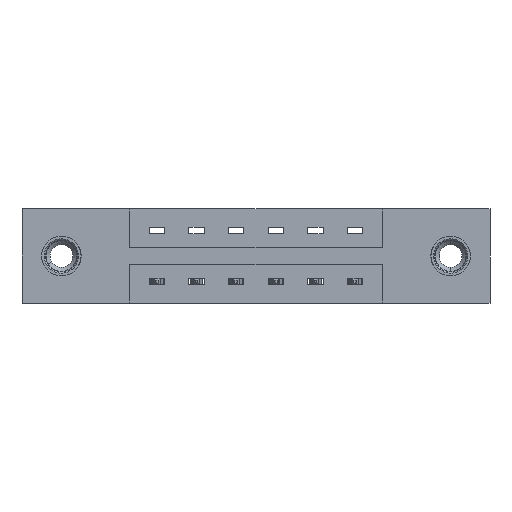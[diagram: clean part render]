
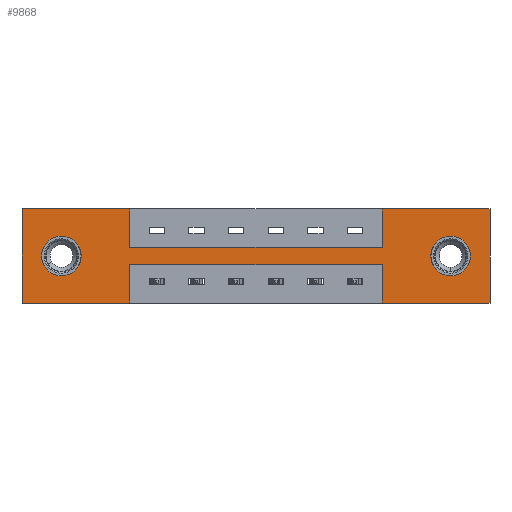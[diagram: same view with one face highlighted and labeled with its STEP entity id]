
A CAD part, front view. The second image highlights one B-rep face of the part: STEP entity #9868.
In plain terms, the highlighted planar face has unit normal (0, -1, 0).
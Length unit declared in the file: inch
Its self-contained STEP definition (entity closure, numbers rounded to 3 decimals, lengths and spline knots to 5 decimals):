
#16 = EDGE_CURVE ( 'NONE', #8204, #5925, #8514, .T. ) ;
#119 = DIRECTION ( 'NONE',  ( 0., 0., -1. ) ) ;
#130 = VERTEX_POINT ( 'NONE', #5805 ) ;
#189 = ORIENTED_EDGE ( 'NONE', *, *, #2319, .F. ) ;
#256 = DIRECTION ( 'NONE',  ( 0., 0., -1. ) ) ;
#269 = LINE ( 'NONE', #8182, #2256 ) ;
#465 = ORIENTED_EDGE ( 'NONE', *, *, #6879, .F. ) ;
#544 = AXIS2_PLACEMENT_3D ( 'NONE', #9028, #4375, #9754 ) ;
#551 = VERTEX_POINT ( 'NONE', #1400 ) ;
#689 = EDGE_LOOP ( 'NONE', ( #8340, #10272, #4398, #189, #2454, #465, #2722, #9022, #719, #7249, #9243, #988 ) ) ;
#719 = ORIENTED_EDGE ( 'NONE', *, *, #2528, .F. ) ;
#733 = LINE ( 'NONE', #8028, #8801 ) ;
#818 = VERTEX_POINT ( 'NONE', #6511 ) ;
#921 = VERTEX_POINT ( 'NONE', #7230 ) ;
#923 = PLANE ( 'NONE',  #8842 ) ;
#988 = ORIENTED_EDGE ( 'NONE', *, *, #16, .F. ) ;
#1034 = DIRECTION ( 'NONE',  ( 0., 1., 0. ) ) ;
#1042 = DIRECTION ( 'NONE',  ( 1., 0., 0. ) ) ;
#1070 = LINE ( 'NONE', #3638, #7321 ) ;
#1096 = DIRECTION ( 'NONE',  ( 0., 0., -1. ) ) ;
#1184 = CARTESIAN_POINT ( 'NONE',  ( 0.425, 0., -0.15 ) ) ;
#1239 = EDGE_CURVE ( 'NONE', #4260, #7239, #8824, .T. ) ;
#1400 = CARTESIAN_POINT ( 'NONE',  ( 0.155, 0., -0.107 ) ) ;
#1656 = DIRECTION ( 'NONE',  ( 0., 0., -1. ) ) ;
#1666 = EDGE_LOOP ( 'NONE', ( #8105, #7600 ) ) ;
#1670 = VECTOR ( 'NONE', #256, 39.37008 ) ;
#1675 = AXIS2_PLACEMENT_3D ( 'NONE', #5954, #1034, #6764 ) ;
#1773 = DIRECTION ( 'NONE',  ( 0., 0., -1. ) ) ;
#1866 = CARTESIAN_POINT ( 'NONE',  ( 1.842, 0., 0. ) ) ;
#1872 = VECTOR ( 'NONE', #8496, 39.37008 ) ;
#1880 = DIRECTION ( 'NONE',  ( 0., 0., -1. ) ) ;
#1893 = CARTESIAN_POINT ( 'NONE',  ( 0., 0., -0.37 ) ) ;
#2256 = VECTOR ( 'NONE', #4251, 39.37008 ) ;
#2319 = EDGE_CURVE ( 'NONE', #818, #4869, #4918, .T. ) ;
#2454 = ORIENTED_EDGE ( 'NONE', *, *, #5068, .F. ) ;
#2528 = EDGE_CURVE ( 'NONE', #7880, #9551, #7389, .T. ) ;
#2550 = CARTESIAN_POINT ( 'NONE',  ( 0.425, 0., -0.22 ) ) ;
#2722 = ORIENTED_EDGE ( 'NONE', *, *, #4743, .F. ) ;
#2820 = CARTESIAN_POINT ( 'NONE',  ( 0., 0., 0. ) ) ;
#2867 = CIRCLE ( 'NONE', #5391, 0.078 ) ;
#2907 = CARTESIAN_POINT ( 'NONE',  ( 0.425, 0., 0. ) ) ;
#2940 = CARTESIAN_POINT ( 'NONE',  ( 1.417, 0., 0. ) ) ;
#3068 = DIRECTION ( 'NONE',  ( -1., 0., 0. ) ) ;
#3164 = EDGE_CURVE ( 'NONE', #8799, #7880, #10157, .T. ) ;
#3201 = LINE ( 'NONE', #10294, #5108 ) ;
#3638 = CARTESIAN_POINT ( 'NONE',  ( 1.417, 0., -0.37 ) ) ;
#3680 = EDGE_CURVE ( 'NONE', #9551, #921, #4774, .T. ) ;
#3857 = CIRCLE ( 'NONE', #544, 0.078 ) ;
#3888 = CARTESIAN_POINT ( 'NONE',  ( 0.155, 0., -0.263 ) ) ;
#4101 = FACE_BOUND ( 'NONE', #8765, .T. ) ;
#4143 = VERTEX_POINT ( 'NONE', #10268 ) ;
#4235 = DIRECTION ( 'NONE',  ( -1., 0., 0. ) ) ;
#4251 = DIRECTION ( 'NONE',  ( -1., 0., 0. ) ) ;
#4260 = VERTEX_POINT ( 'NONE', #4265 ) ;
#4265 = CARTESIAN_POINT ( 'NONE',  ( 1.687, 0., -0.263 ) ) ;
#4375 = DIRECTION ( 'NONE',  ( 0., 1., 0. ) ) ;
#4398 = ORIENTED_EDGE ( 'NONE', *, *, #5270, .F. ) ;
#4439 = CARTESIAN_POINT ( 'NONE',  ( 0.425, 0., 0. ) ) ;
#4598 = FACE_BOUND ( 'NONE', #1666, .T. ) ;
#4679 = LINE ( 'NONE', #5234, #1670 ) ;
#4743 = EDGE_CURVE ( 'NONE', #921, #4143, #5968, .T. ) ;
#4774 = LINE ( 'NONE', #8308, #8216 ) ;
#4869 = VERTEX_POINT ( 'NONE', #5518 ) ;
#4918 = LINE ( 'NONE', #5027, #8817 ) ;
#5027 = CARTESIAN_POINT ( 'NONE',  ( 0., 0., -0.37 ) ) ;
#5068 = EDGE_CURVE ( 'NONE', #8458, #818, #3201, .T. ) ;
#5108 = VECTOR ( 'NONE', #1656, 39.37008 ) ;
#5120 = DIRECTION ( 'NONE',  ( 0., 1., 0. ) ) ;
#5234 = CARTESIAN_POINT ( 'NONE',  ( 0.425, 0., -0.37 ) ) ;
#5270 = EDGE_CURVE ( 'NONE', #4869, #130, #1070, .T. ) ;
#5391 = AXIS2_PLACEMENT_3D ( 'NONE', #9713, #5120, #119 ) ;
#5477 = VERTEX_POINT ( 'NONE', #3888 ) ;
#5518 = CARTESIAN_POINT ( 'NONE',  ( 1.417, 0., -0.37 ) ) ;
#5701 = CIRCLE ( 'NONE', #1675, 0.078 ) ;
#5785 = EDGE_CURVE ( 'NONE', #130, #8848, #269, .T. ) ;
#5805 = CARTESIAN_POINT ( 'NONE',  ( 1.417, 0., -0.22 ) ) ;
#5925 = VERTEX_POINT ( 'NONE', #1893 ) ;
#5939 = AXIS2_PLACEMENT_3D ( 'NONE', #9605, #6271, #1880 ) ;
#5954 = CARTESIAN_POINT ( 'NONE',  ( 0.155, 0., -0.185 ) ) ;
#5968 = LINE ( 'NONE', #2940, #1872 ) ;
#6022 = VECTOR ( 'NONE', #7617, 39.37008 ) ;
#6063 = ORIENTED_EDGE ( 'NONE', *, *, #7382, .T. ) ;
#6144 = VECTOR ( 'NONE', #8409, 39.37008 ) ;
#6246 = ORIENTED_EDGE ( 'NONE', *, *, #1239, .T. ) ;
#6271 = DIRECTION ( 'NONE',  ( 0., 1., 0. ) ) ;
#6434 = VECTOR ( 'NONE', #3068, 39.37008 ) ;
#6511 = CARTESIAN_POINT ( 'NONE',  ( 1.842, 0., -0.37 ) ) ;
#6656 = DIRECTION ( 'NONE',  ( 0., -1., 0. ) ) ;
#6764 = DIRECTION ( 'NONE',  ( 0., 0., 1. ) ) ;
#6862 = EDGE_CURVE ( 'NONE', #8848, #8204, #4679, .T. ) ;
#6879 = EDGE_CURVE ( 'NONE', #4143, #8458, #9835, .T. ) ;
#7197 = EDGE_CURVE ( 'NONE', #5925, #8799, #733, .T. ) ;
#7230 = CARTESIAN_POINT ( 'NONE',  ( 1.417, 0., -0.15 ) ) ;
#7239 = VERTEX_POINT ( 'NONE', #10258 ) ;
#7249 = ORIENTED_EDGE ( 'NONE', *, *, #3164, .F. ) ;
#7321 = VECTOR ( 'NONE', #9815, 39.37008 ) ;
#7382 = EDGE_CURVE ( 'NONE', #7239, #4260, #2867, .T. ) ;
#7389 = LINE ( 'NONE', #4439, #9377 ) ;
#7600 = ORIENTED_EDGE ( 'NONE', *, *, #9943, .T. ) ;
#7617 = DIRECTION ( 'NONE',  ( 1., 0., 0. ) ) ;
#7880 = VERTEX_POINT ( 'NONE', #2907 ) ;
#8028 = CARTESIAN_POINT ( 'NONE',  ( 0., 0., 0. ) ) ;
#8092 = CARTESIAN_POINT ( 'NONE',  ( 0., 0., 0. ) ) ;
#8105 = ORIENTED_EDGE ( 'NONE', *, *, #9931, .T. ) ;
#8182 = CARTESIAN_POINT ( 'NONE',  ( 0.425, 0., -0.22 ) ) ;
#8204 = VERTEX_POINT ( 'NONE', #10236 ) ;
#8216 = VECTOR ( 'NONE', #1042, 39.37008 ) ;
#8290 = FACE_OUTER_BOUND ( 'NONE', #689, .T. ) ;
#8308 = CARTESIAN_POINT ( 'NONE',  ( 0.425, 0., -0.15 ) ) ;
#8340 = ORIENTED_EDGE ( 'NONE', *, *, #6862, .F. ) ;
#8409 = DIRECTION ( 'NONE',  ( 1., 0., 0. ) ) ;
#8458 = VERTEX_POINT ( 'NONE', #1866 ) ;
#8496 = DIRECTION ( 'NONE',  ( 0., 0., 1. ) ) ;
#8514 = LINE ( 'NONE', #8919, #6434 ) ;
#8764 = DIRECTION ( 'NONE',  ( 0., 0., 1. ) ) ;
#8765 = EDGE_LOOP ( 'NONE', ( #6063, #6246 ) ) ;
#8799 = VERTEX_POINT ( 'NONE', #8092 ) ;
#8801 = VECTOR ( 'NONE', #8764, 39.37008 ) ;
#8817 = VECTOR ( 'NONE', #4235, 39.37008 ) ;
#8824 = CIRCLE ( 'NONE', #5939, 0.078 ) ;
#8842 = AXIS2_PLACEMENT_3D ( 'NONE', #9658, #6656, #1773 ) ;
#8848 = VERTEX_POINT ( 'NONE', #2550 ) ;
#8919 = CARTESIAN_POINT ( 'NONE',  ( 0., 0., -0.37 ) ) ;
#9022 = ORIENTED_EDGE ( 'NONE', *, *, #3680, .F. ) ;
#9028 = CARTESIAN_POINT ( 'NONE',  ( 0.155, 0., -0.185 ) ) ;
#9129 = CARTESIAN_POINT ( 'NONE',  ( 0., 0., 0. ) ) ;
#9243 = ORIENTED_EDGE ( 'NONE', *, *, #7197, .F. ) ;
#9377 = VECTOR ( 'NONE', #1096, 39.37008 ) ;
#9551 = VERTEX_POINT ( 'NONE', #1184 ) ;
#9605 = CARTESIAN_POINT ( 'NONE',  ( 1.687, 0., -0.185 ) ) ;
#9658 = CARTESIAN_POINT ( 'NONE',  ( 0., 0., -0.37 ) ) ;
#9713 = CARTESIAN_POINT ( 'NONE',  ( 1.687, 0., -0.185 ) ) ;
#9754 = DIRECTION ( 'NONE',  ( 0., 0., 1. ) ) ;
#9815 = DIRECTION ( 'NONE',  ( 0., 0., 1. ) ) ;
#9835 = LINE ( 'NONE', #2820, #6022 ) ;
#9868 = ADVANCED_FACE ( 'NONE', ( #4101, #4598, #8290 ), #923, .T. ) ;
#9931 = EDGE_CURVE ( 'NONE', #551, #5477, #3857, .T. ) ;
#9943 = EDGE_CURVE ( 'NONE', #5477, #551, #5701, .T. ) ;
#10157 = LINE ( 'NONE', #9129, #6144 ) ;
#10236 = CARTESIAN_POINT ( 'NONE',  ( 0.425, 0., -0.37 ) ) ;
#10258 = CARTESIAN_POINT ( 'NONE',  ( 1.687, 0., -0.107 ) ) ;
#10268 = CARTESIAN_POINT ( 'NONE',  ( 1.417, 0., 0. ) ) ;
#10272 = ORIENTED_EDGE ( 'NONE', *, *, #5785, .F. ) ;
#10294 = CARTESIAN_POINT ( 'NONE',  ( 1.842, 0., 0. ) ) ;
